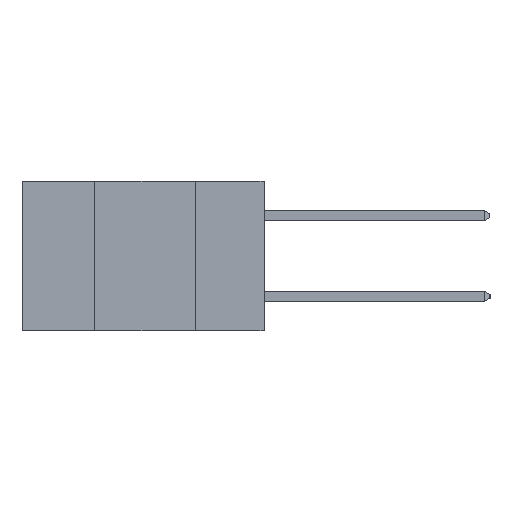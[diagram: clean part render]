
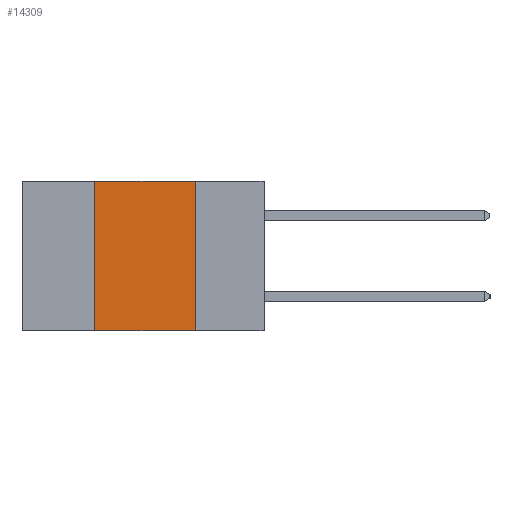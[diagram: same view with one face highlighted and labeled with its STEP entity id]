
A CAD part, left-side view. The second image highlights one B-rep face of the part: STEP entity #14309.
In plain terms, the highlighted planar face has unit normal (-1, 0, 0).
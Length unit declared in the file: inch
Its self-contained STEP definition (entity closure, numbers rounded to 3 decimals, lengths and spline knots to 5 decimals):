
#990 = CARTESIAN_POINT ( 'NONE',  ( 0., 0.42, -0.37 ) ) ;
#1184 = VERTEX_POINT ( 'NONE', #7118 ) ;
#1677 = CARTESIAN_POINT ( 'NONE',  ( 0., 0.42, 0. ) ) ;
#3237 = VERTEX_POINT ( 'NONE', #1677 ) ;
#3746 = VERTEX_POINT ( 'NONE', #19795 ) ;
#3980 = ORIENTED_EDGE ( 'NONE', *, *, #19416, .F. ) ;
#4865 = VECTOR ( 'NONE', #7845, 39.37008 ) ;
#5214 = LINE ( 'NONE', #6263, #17121 ) ;
#5385 = LINE ( 'NONE', #9401, #4865 ) ;
#5868 = EDGE_CURVE ( 'NONE', #3237, #3746, #11620, .T. ) ;
#6263 = CARTESIAN_POINT ( 'NONE',  ( 0., 0.6, -0.37 ) ) ;
#6328 = VERTEX_POINT ( 'NONE', #12629 ) ;
#6365 = DIRECTION ( 'NONE',  ( 1., 0., 0. ) ) ;
#7118 = CARTESIAN_POINT ( 'NONE',  ( 0., 0.42, -0.37 ) ) ;
#7357 = VECTOR ( 'NONE', #19695, 39.37008 ) ;
#7819 = LINE ( 'NONE', #990, #7357 ) ;
#7845 = DIRECTION ( 'NONE',  ( 0., 0., -1. ) ) ;
#8079 = EDGE_CURVE ( 'NONE', #1184, #3237, #7819, .T. ) ;
#8149 = ORIENTED_EDGE ( 'NONE', *, *, #5868, .F. ) ;
#8625 = ORIENTED_EDGE ( 'NONE', *, *, #8079, .F. ) ;
#9401 = CARTESIAN_POINT ( 'NONE',  ( 0., 0.17, -0.37 ) ) ;
#9473 = CARTESIAN_POINT ( 'NONE',  ( 0., 0.6, 0. ) ) ;
#11263 = EDGE_CURVE ( 'NONE', #1184, #6328, #5214, .T. ) ;
#11620 = LINE ( 'NONE', #9473, #15700 ) ;
#12629 = CARTESIAN_POINT ( 'NONE',  ( 0., 0.17, -0.37 ) ) ;
#12827 = ORIENTED_EDGE ( 'NONE', *, *, #11263, .T. ) ;
#14167 = PLANE ( 'NONE',  #16472 ) ;
#14208 = DIRECTION ( 'NONE',  ( 0., -1., 0. ) ) ;
#14309 = ADVANCED_FACE ( 'NONE', ( #14396 ), #14167, .F. ) ;
#14396 = FACE_OUTER_BOUND ( 'NONE', #17031, .T. ) ;
#15534 = DIRECTION ( 'NONE',  ( 0., -1., 0. ) ) ;
#15700 = VECTOR ( 'NONE', #14208, 39.37008 ) ;
#16472 = AXIS2_PLACEMENT_3D ( 'NONE', #17141, #6365, #17202 ) ;
#17031 = EDGE_LOOP ( 'NONE', ( #3980, #8149, #8625, #12827 ) ) ;
#17121 = VECTOR ( 'NONE', #15534, 39.37008 ) ;
#17141 = CARTESIAN_POINT ( 'NONE',  ( 0., 0.6, 0. ) ) ;
#17202 = DIRECTION ( 'NONE',  ( 0., 0., -1. ) ) ;
#19416 = EDGE_CURVE ( 'NONE', #3746, #6328, #5385, .T. ) ;
#19695 = DIRECTION ( 'NONE',  ( 0., 0., 1. ) ) ;
#19795 = CARTESIAN_POINT ( 'NONE',  ( 0., 0.17, 0. ) ) ;
